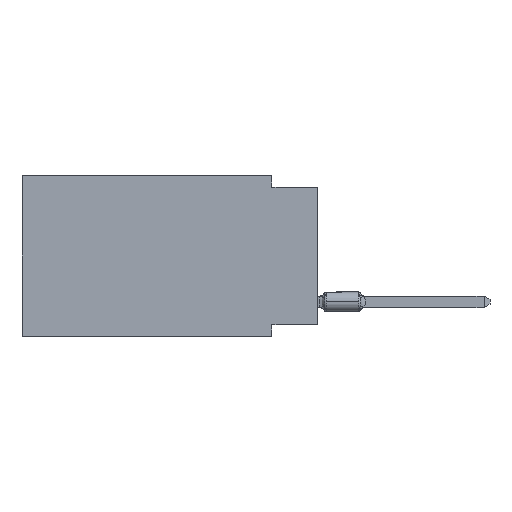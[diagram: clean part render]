
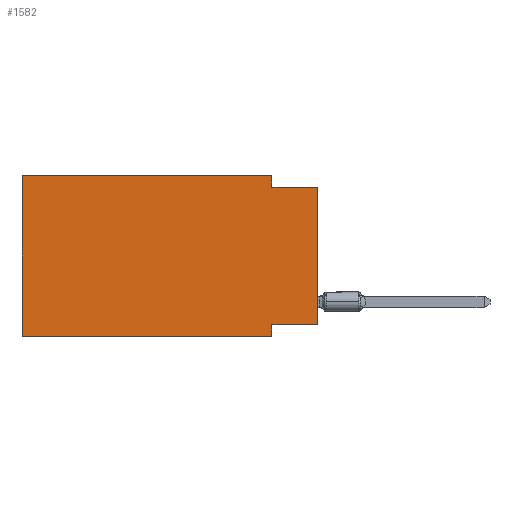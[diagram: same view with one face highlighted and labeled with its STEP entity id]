
A CAD part, left-side view. The second image highlights one B-rep face of the part: STEP entity #1582.
In plain terms, the highlighted planar face has unit normal (-1, 0, 0).
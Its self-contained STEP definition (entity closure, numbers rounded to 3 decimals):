
#110 = DIRECTION ( 'NONE',  ( 0., 0., 1. ) ) ;
#239 = CARTESIAN_POINT ( 'NONE',  ( 0., 16.383, 0. ) ) ;
#470 = VERTEX_POINT ( 'NONE', #6016 ) ;
#500 = EDGE_CURVE ( 'NONE', #10879, #6866, #15472, .T. ) ;
#670 = FACE_OUTER_BOUND ( 'NONE', #19167, .T. ) ;
#1138 = VECTOR ( 'NONE', #19700, 1000. ) ;
#1150 = EDGE_CURVE ( 'NONE', #3348, #14753, #6614, .T. ) ;
#1452 = ORIENTED_EDGE ( 'NONE', *, *, #10876, .F. ) ;
#1582 = ADVANCED_FACE ( 'NONE', ( #670 ), #19956, .F. ) ;
#1788 = DIRECTION ( 'NONE',  ( 0., 1., 0. ) ) ;
#2324 = LINE ( 'NONE', #20443, #7000 ) ;
#3178 = LINE ( 'NONE', #16492, #14869 ) ;
#3188 = ORIENTED_EDGE ( 'NONE', *, *, #12450, .F. ) ;
#3348 = VERTEX_POINT ( 'NONE', #5488 ) ;
#4524 = EDGE_CURVE ( 'NONE', #7235, #6866, #6797, .T. ) ;
#4953 = ORIENTED_EDGE ( 'NONE', *, *, #10430, .T. ) ;
#5488 = CARTESIAN_POINT ( 'NONE',  ( 0., 16.383, 0. ) ) ;
#5521 = LINE ( 'NONE', #16881, #16353 ) ;
#5676 = EDGE_CURVE ( 'NONE', #470, #8138, #5521, .T. ) ;
#5709 = CARTESIAN_POINT ( 'NONE',  ( 0., 2.54, -8.89 ) ) ;
#6016 = CARTESIAN_POINT ( 'NONE',  ( 0., 2.54, -0.635 ) ) ;
#6614 = LINE ( 'NONE', #13158, #1138 ) ;
#6797 = LINE ( 'NONE', #11948, #16937 ) ;
#6866 = VERTEX_POINT ( 'NONE', #10089 ) ;
#7000 = VECTOR ( 'NONE', #15515, 1000. ) ;
#7203 = DIRECTION ( 'NONE',  ( 1., 0., 0. ) ) ;
#7235 = VERTEX_POINT ( 'NONE', #10104 ) ;
#7258 = EDGE_CURVE ( 'NONE', #7235, #3348, #10215, .T. ) ;
#7314 = AXIS2_PLACEMENT_3D ( 'NONE', #239, #7203, #18227 ) ;
#7487 = CARTESIAN_POINT ( 'NONE',  ( 0., 0., -0.635 ) ) ;
#8066 = VERTEX_POINT ( 'NONE', #16816 ) ;
#8138 = VERTEX_POINT ( 'NONE', #7487 ) ;
#8421 = ORIENTED_EDGE ( 'NONE', *, *, #7258, .F. ) ;
#8732 = DIRECTION ( 'NONE',  ( 0., -1., 0. ) ) ;
#10089 = CARTESIAN_POINT ( 'NONE',  ( 0., 2.54, -8.89 ) ) ;
#10104 = CARTESIAN_POINT ( 'NONE',  ( 0., 16.383, -8.89 ) ) ;
#10215 = LINE ( 'NONE', #16760, #20067 ) ;
#10430 = EDGE_CURVE ( 'NONE', #8066, #8138, #21136, .T. ) ;
#10876 = EDGE_CURVE ( 'NONE', #14753, #470, #2324, .T. ) ;
#10879 = VERTEX_POINT ( 'NONE', #18717 ) ;
#11948 = CARTESIAN_POINT ( 'NONE',  ( 0., 16.383, -8.89 ) ) ;
#12450 = EDGE_CURVE ( 'NONE', #8066, #10879, #3178, .T. ) ;
#13085 = CARTESIAN_POINT ( 'NONE',  ( 0., 0., 0. ) ) ;
#13158 = CARTESIAN_POINT ( 'NONE',  ( 0., 16.383, 0. ) ) ;
#14753 = VERTEX_POINT ( 'NONE', #18501 ) ;
#14869 = VECTOR ( 'NONE', #1788, 1000. ) ;
#15139 = VECTOR ( 'NONE', #15582, 1000. ) ;
#15472 = LINE ( 'NONE', #5709, #15139 ) ;
#15515 = DIRECTION ( 'NONE',  ( 0., 0., -1. ) ) ;
#15582 = DIRECTION ( 'NONE',  ( 0., 0., -1. ) ) ;
#15710 = DIRECTION ( 'NONE',  ( 0., 0., 1. ) ) ;
#16353 = VECTOR ( 'NONE', #8732, 1000. ) ;
#16492 = CARTESIAN_POINT ( 'NONE',  ( 0., 0., -8.255 ) ) ;
#16524 = ORIENTED_EDGE ( 'NONE', *, *, #5676, .F. ) ;
#16760 = CARTESIAN_POINT ( 'NONE',  ( 0., 16.383, 0. ) ) ;
#16816 = CARTESIAN_POINT ( 'NONE',  ( 0., 0., -8.255 ) ) ;
#16881 = CARTESIAN_POINT ( 'NONE',  ( 0., 0., -0.635 ) ) ;
#16937 = VECTOR ( 'NONE', #20101, 1000. ) ;
#17039 = ORIENTED_EDGE ( 'NONE', *, *, #500, .F. ) ;
#17097 = ORIENTED_EDGE ( 'NONE', *, *, #1150, .F. ) ;
#18227 = DIRECTION ( 'NONE',  ( 0., 0., -1. ) ) ;
#18501 = CARTESIAN_POINT ( 'NONE',  ( 0., 2.54, 0. ) ) ;
#18717 = CARTESIAN_POINT ( 'NONE',  ( 0., 2.54, -8.255 ) ) ;
#18971 = VECTOR ( 'NONE', #110, 1000. ) ;
#19065 = ORIENTED_EDGE ( 'NONE', *, *, #4524, .T. ) ;
#19167 = EDGE_LOOP ( 'NONE', ( #4953, #16524, #1452, #17097, #8421, #19065, #17039, #3188 ) ) ;
#19700 = DIRECTION ( 'NONE',  ( 0., -1., 0. ) ) ;
#19956 = PLANE ( 'NONE',  #7314 ) ;
#20067 = VECTOR ( 'NONE', #15710, 1000. ) ;
#20101 = DIRECTION ( 'NONE',  ( 0., -1., 0. ) ) ;
#20443 = CARTESIAN_POINT ( 'NONE',  ( 0., 2.54, 0. ) ) ;
#21136 = LINE ( 'NONE', #13085, #18971 ) ;
